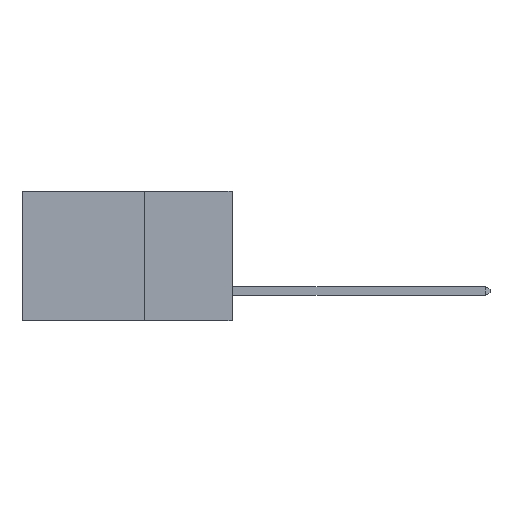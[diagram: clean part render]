
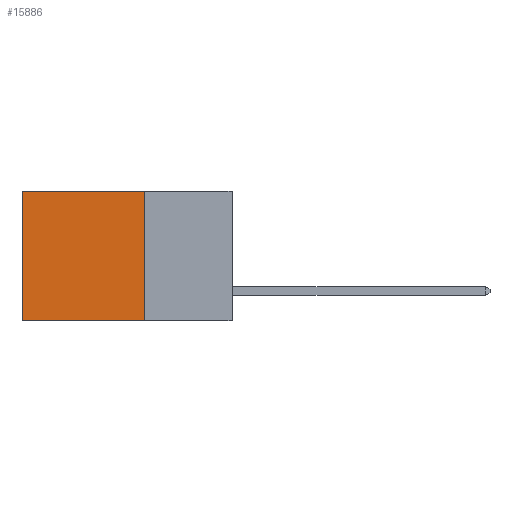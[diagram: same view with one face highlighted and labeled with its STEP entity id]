
A CAD part, left-side view. The second image highlights one B-rep face of the part: STEP entity #15886.
In plain terms, the highlighted planar face has unit normal (-1, 0, 0).
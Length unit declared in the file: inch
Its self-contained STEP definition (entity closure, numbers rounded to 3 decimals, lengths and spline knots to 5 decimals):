
#292 = DIRECTION ( 'NONE',  ( 0., 0., -1. ) ) ;
#691 = EDGE_CURVE ( 'NONE', #5531, #20619, #22988, .T. ) ;
#1286 = CARTESIAN_POINT ( 'NONE',  ( 0.2875, 0.25, 0. ) ) ;
#1664 = DIRECTION ( 'NONE',  ( 0., 0., -1. ) ) ;
#1840 = DIRECTION ( 'NONE',  ( 0., 1., 0. ) ) ;
#2999 = CARTESIAN_POINT ( 'NONE',  ( 0.2875, 0.25, 0. ) ) ;
#4046 = EDGE_CURVE ( 'NONE', #5531, #21117, #12326, .T. ) ;
#4242 = ORIENTED_EDGE ( 'NONE', *, *, #4046, .T. ) ;
#5139 = VERTEX_POINT ( 'NONE', #8389 ) ;
#5319 = CARTESIAN_POINT ( 'NONE',  ( 0.2875, 0.25, 0. ) ) ;
#5531 = VERTEX_POINT ( 'NONE', #24386 ) ;
#6491 = EDGE_CURVE ( 'NONE', #21117, #5139, #9894, .T. ) ;
#7319 = DIRECTION ( 'NONE',  ( 0., 0., -1. ) ) ;
#8321 = CARTESIAN_POINT ( 'NONE',  ( 0.2875, 0.6, 0. ) ) ;
#8325 = EDGE_CURVE ( 'NONE', #20619, #5139, #19309, .T. ) ;
#8389 = CARTESIAN_POINT ( 'NONE',  ( 0.2875, 0.6, -0.37 ) ) ;
#8880 = ORIENTED_EDGE ( 'NONE', *, *, #6491, .T. ) ;
#9224 = PLANE ( 'NONE',  #23930 ) ;
#9283 = VECTOR ( 'NONE', #292, 39.37008 ) ;
#9364 = VECTOR ( 'NONE', #1840, 39.37008 ) ;
#9894 = LINE ( 'NONE', #8321, #9283 ) ;
#9933 = FACE_OUTER_BOUND ( 'NONE', #13664, .T. ) ;
#12326 = LINE ( 'NONE', #2999, #16683 ) ;
#13031 = ORIENTED_EDGE ( 'NONE', *, *, #691, .F. ) ;
#13079 = VECTOR ( 'NONE', #1664, 39.37008 ) ;
#13664 = EDGE_LOOP ( 'NONE', ( #8880, #24446, #13031, #4242 ) ) ;
#15886 = ADVANCED_FACE ( 'NONE', ( #9933 ), #9224, .F. ) ;
#16683 = VECTOR ( 'NONE', #20269, 39.37008 ) ;
#17495 = CARTESIAN_POINT ( 'NONE',  ( 0.2875, 0.6, 0. ) ) ;
#18623 = DIRECTION ( 'NONE',  ( 1., 0., 0. ) ) ;
#19309 = LINE ( 'NONE', #22923, #9364 ) ;
#20269 = DIRECTION ( 'NONE',  ( 0., 1., 0. ) ) ;
#20619 = VERTEX_POINT ( 'NONE', #23436 ) ;
#21117 = VERTEX_POINT ( 'NONE', #17495 ) ;
#22923 = CARTESIAN_POINT ( 'NONE',  ( 0.2875, 0.25, -0.37 ) ) ;
#22988 = LINE ( 'NONE', #1286, #13079 ) ;
#23436 = CARTESIAN_POINT ( 'NONE',  ( 0.2875, 0.25, -0.37 ) ) ;
#23930 = AXIS2_PLACEMENT_3D ( 'NONE', #5319, #18623, #7319 ) ;
#24386 = CARTESIAN_POINT ( 'NONE',  ( 0.2875, 0.25, 0. ) ) ;
#24446 = ORIENTED_EDGE ( 'NONE', *, *, #8325, .F. ) ;
